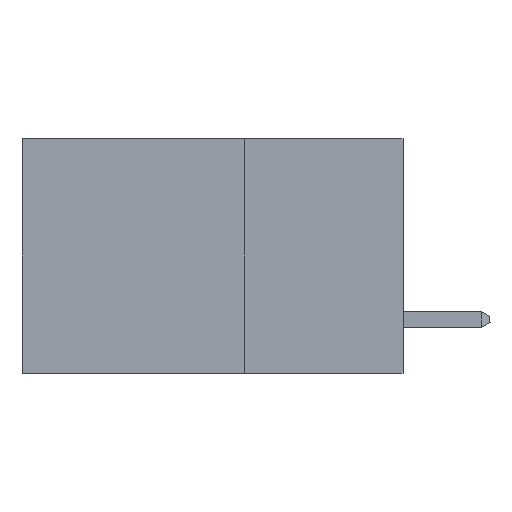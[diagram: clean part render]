
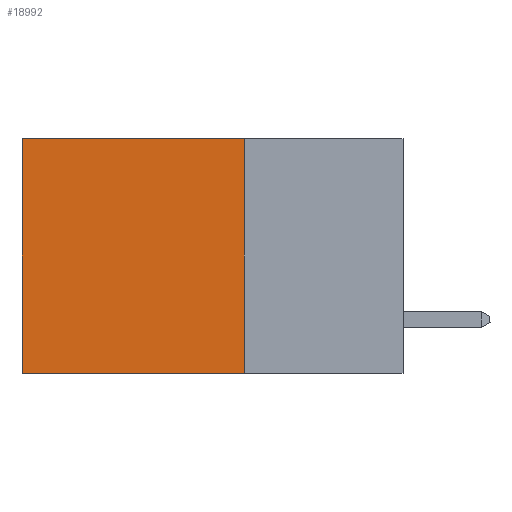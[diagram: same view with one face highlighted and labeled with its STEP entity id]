
A CAD part, left-side view. The second image highlights one B-rep face of the part: STEP entity #18992.
In plain terms, the highlighted planar face has unit normal (-1, 0, 0).
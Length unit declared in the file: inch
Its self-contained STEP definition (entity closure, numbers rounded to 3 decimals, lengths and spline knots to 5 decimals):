
#128 = DIRECTION ( 'NONE',  ( 0., 1., 0. ) ) ;
#3539 = DIRECTION ( 'NONE',  ( 0., 0., -1. ) ) ;
#3994 = ORIENTED_EDGE ( 'NONE', *, *, #27196, .F. ) ;
#4115 = VECTOR ( 'NONE', #128, 39.37008 ) ;
#4244 = LINE ( 'NONE', #13784, #31971 ) ;
#4354 = DIRECTION ( 'NONE',  ( 0., 0., -1. ) ) ;
#4372 = ORIENTED_EDGE ( 'NONE', *, *, #4863, .F. ) ;
#4863 = EDGE_CURVE ( 'NONE', #24699, #12014, #9896, .T. ) ;
#5190 = VECTOR ( 'NONE', #21191, 39.37008 ) ;
#5941 = CARTESIAN_POINT ( 'NONE',  ( 0.2875, 0.25, -0.37 ) ) ;
#8177 = CARTESIAN_POINT ( 'NONE',  ( 0.2875, 0.25, 0. ) ) ;
#8229 = AXIS2_PLACEMENT_3D ( 'NONE', #21955, #29583, #14393 ) ;
#9491 = VERTEX_POINT ( 'NONE', #12666 ) ;
#9896 = LINE ( 'NONE', #8177, #22598 ) ;
#11709 = LINE ( 'NONE', #17985, #4115 ) ;
#12014 = VERTEX_POINT ( 'NONE', #15906 ) ;
#12149 = EDGE_CURVE ( 'NONE', #29466, #9491, #4244, .T. ) ;
#12666 = CARTESIAN_POINT ( 'NONE',  ( 0.2875, 0.6, -0.37 ) ) ;
#13784 = CARTESIAN_POINT ( 'NONE',  ( 0.2875, 0.6, 0. ) ) ;
#14290 = PLANE ( 'NONE',  #8229 ) ;
#14393 = DIRECTION ( 'NONE',  ( 0., 0., -1. ) ) ;
#15654 = EDGE_LOOP ( 'NONE', ( #26772, #3994, #4372, #32862 ) ) ;
#15906 = CARTESIAN_POINT ( 'NONE',  ( 0.2875, 0.25, -0.37 ) ) ;
#17985 = CARTESIAN_POINT ( 'NONE',  ( 0.2875, 0.25, 0. ) ) ;
#18992 = ADVANCED_FACE ( 'NONE', ( #27708 ), #14290, .F. ) ;
#21191 = DIRECTION ( 'NONE',  ( 0., 1., 0. ) ) ;
#21955 = CARTESIAN_POINT ( 'NONE',  ( 0.2875, 0.25, 0. ) ) ;
#22598 = VECTOR ( 'NONE', #4354, 39.37008 ) ;
#23911 = LINE ( 'NONE', #5941, #5190 ) ;
#24699 = VERTEX_POINT ( 'NONE', #31877 ) ;
#25296 = CARTESIAN_POINT ( 'NONE',  ( 0.2875, 0.6, 0. ) ) ;
#26772 = ORIENTED_EDGE ( 'NONE', *, *, #12149, .T. ) ;
#27196 = EDGE_CURVE ( 'NONE', #12014, #9491, #23911, .T. ) ;
#27708 = FACE_OUTER_BOUND ( 'NONE', #15654, .T. ) ;
#29466 = VERTEX_POINT ( 'NONE', #25296 ) ;
#29539 = EDGE_CURVE ( 'NONE', #24699, #29466, #11709, .T. ) ;
#29583 = DIRECTION ( 'NONE',  ( 1., 0., 0. ) ) ;
#31877 = CARTESIAN_POINT ( 'NONE',  ( 0.2875, 0.25, 0. ) ) ;
#31971 = VECTOR ( 'NONE', #3539, 39.37008 ) ;
#32862 = ORIENTED_EDGE ( 'NONE', *, *, #29539, .T. ) ;
